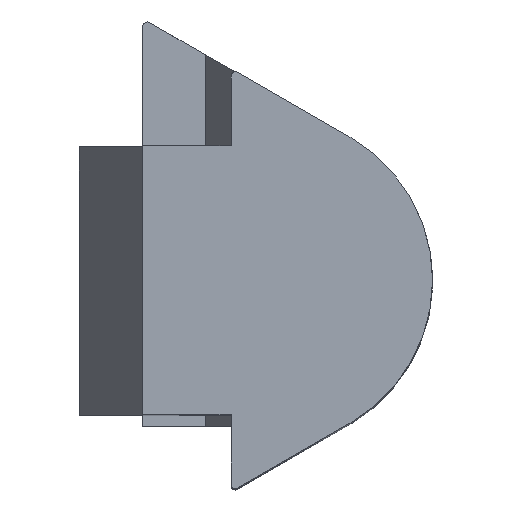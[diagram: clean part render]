
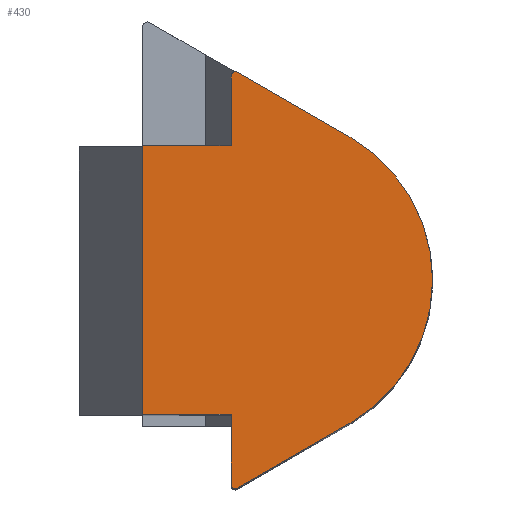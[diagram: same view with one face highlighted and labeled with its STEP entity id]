
A CAD part, top view. The second image highlights one B-rep face of the part: STEP entity #430.
In plain terms, the highlighted planar face has unit normal (0, 0, 1).
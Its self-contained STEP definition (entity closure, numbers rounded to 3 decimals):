
#4 = DIRECTION ( 'NONE',  ( -0.866, -0.5, 0. ) ) ;
#23 = ORIENTED_EDGE ( 'NONE', *, *, #490, .F. ) ;
#28 = LINE ( 'NONE', #186, #461 ) ;
#29 = AXIS2_PLACEMENT_3D ( 'NONE', #381, #360, #355 ) ;
#31 = DIRECTION ( 'NONE',  ( 0., -1., 0. ) ) ;
#33 = DIRECTION ( 'NONE',  ( 0., -1., 0. ) ) ;
#35 = CARTESIAN_POINT ( 'NONE',  ( 2.242, 1.045, -2.686 ) ) ;
#55 = VERTEX_POINT ( 'NONE', #818 ) ;
#66 = AXIS2_PLACEMENT_3D ( 'NONE', #272, #269, #264 ) ;
#73 = ORIENTED_EDGE ( 'NONE', *, *, #546, .F. ) ;
#75 = AXIS2_PLACEMENT_3D ( 'NONE', #684, #641, #633 ) ;
#81 = CARTESIAN_POINT ( 'NONE',  ( 2.306, -2.942, -2.686 ) ) ;
#88 = CARTESIAN_POINT ( 'NONE',  ( 3.958, -2.062, -2.686 ) ) ;
#89 = VECTOR ( 'NONE', #289, 1000. ) ;
#104 = VERTEX_POINT ( 'NONE', #437 ) ;
#109 = CARTESIAN_POINT ( 'NONE',  ( 3.958, -2.062, -2.686 ) ) ;
#111 = DIRECTION ( 'NONE',  ( -1., 0., 0. ) ) ;
#112 = AXIS2_PLACEMENT_3D ( 'NONE', #745, #744, #712 ) ;
#114 = ORIENTED_EDGE ( 'NONE', *, *, #393, .F. ) ;
#117 = AXIS2_PLACEMENT_3D ( 'NONE', #911, #908, #906 ) ;
#128 = CARTESIAN_POINT ( 'NONE',  ( 2.242, -1.045, -2.686 ) ) ;
#132 = CARTESIAN_POINT ( 'NONE',  ( 2.102, 1.937, -2.686 ) ) ;
#139 = AXIS2_PLACEMENT_3D ( 'NONE', #81, #973, #968 ) ;
#141 = CARTESIAN_POINT ( 'NONE',  ( 2.242, 1.937, -2.686 ) ) ;
#156 = DIRECTION ( 'NONE',  ( 0., 1., 0. ) ) ;
#186 = CARTESIAN_POINT ( 'NONE',  ( 0.972, -2.089, -2.686 ) ) ;
#223 = VECTOR ( 'NONE', #33, 1000. ) ;
#224 = ORIENTED_EDGE ( 'NONE', *, *, #370, .F. ) ;
#256 = LINE ( 'NONE', #88, #671 ) ;
#264 = DIRECTION ( 'NONE',  ( -0.5, 0.866, 0. ) ) ;
#267 = CARTESIAN_POINT ( 'NONE',  ( 2.102, -1.937, -2.686 ) ) ;
#269 = DIRECTION ( 'NONE',  ( 0., 0., -1. ) ) ;
#272 = CARTESIAN_POINT ( 'NONE',  ( 2.306, 2.942, -2.686 ) ) ;
#279 = EDGE_LOOP ( 'NONE', ( #515, #224, #73, #543, #462, #114, #333, #821, #23, #579, #930, #374 ) ) ;
#289 = DIRECTION ( 'NONE',  ( 1., 0., 0. ) ) ;
#298 = CIRCLE ( 'NONE', #66, 0.063 ) ;
#299 = LINE ( 'NONE', #128, #701 ) ;
#333 = ORIENTED_EDGE ( 'NONE', *, *, #505, .T. ) ;
#336 = DIRECTION ( 'NONE',  ( 0.866, -0.5, 0. ) ) ;
#341 = EDGE_CURVE ( 'NONE', #392, #765, #576, .T. ) ;
#355 = DIRECTION ( 'NONE',  ( 0.5, 0.866, 0. ) ) ;
#360 = DIRECTION ( 'NONE',  ( 0., 0., -1. ) ) ;
#370 = EDGE_CURVE ( 'NONE', #501, #832, #256, .T. ) ;
#374 = ORIENTED_EDGE ( 'NONE', *, *, #380, .F. ) ;
#380 = EDGE_CURVE ( 'NONE', #519, #411, #839, .T. ) ;
#381 = CARTESIAN_POINT ( 'NONE',  ( 2.767, 0., -2.686 ) ) ;
#389 = FACE_OUTER_BOUND ( 'NONE', #279, .T. ) ;
#392 = VERTEX_POINT ( 'NONE', #431 ) ;
#393 = EDGE_CURVE ( 'NONE', #436, #104, #797, .T. ) ;
#411 = VERTEX_POINT ( 'NONE', #812 ) ;
#417 = CIRCLE ( 'NONE', #112, 0.064 ) ;
#420 = EDGE_CURVE ( 'NONE', #832, #519, #417, .T. ) ;
#430 = ADVANCED_FACE ( 'NONE', ( #389 ), #643, .T. ) ;
#431 = CARTESIAN_POINT ( 'NONE',  ( 2.338, 2.997, -2.686 ) ) ;
#436 = VERTEX_POINT ( 'NONE', #578 ) ;
#437 = CARTESIAN_POINT ( 'NONE',  ( 2.274, 2.997, -2.686 ) ) ;
#461 = VECTOR ( 'NONE', #156, 1000. ) ;
#462 = ORIENTED_EDGE ( 'NONE', *, *, #477, .F. ) ;
#477 = EDGE_CURVE ( 'NONE', #104, #392, #298, .T. ) ;
#490 = EDGE_CURVE ( 'NONE', #682, #55, #28, .T. ) ;
#501 = VERTEX_POINT ( 'NONE', #109 ) ;
#505 = EDGE_CURVE ( 'NONE', #436, #673, #630, .T. ) ;
#515 = ORIENTED_EDGE ( 'NONE', *, *, #420, .F. ) ;
#519 = VERTEX_POINT ( 'NONE', #939 ) ;
#524 = VECTOR ( 'NONE', #111, 1000. ) ;
#543 = ORIENTED_EDGE ( 'NONE', *, *, #341, .F. ) ;
#546 = EDGE_CURVE ( 'NONE', #765, #501, #917, .T. ) ;
#558 = EDGE_CURVE ( 'NONE', #673, #55, #896, .T. ) ;
#562 = EDGE_CURVE ( 'NONE', #682, #949, #743, .T. ) ;
#566 = EDGE_CURVE ( 'NONE', #949, #411, #299, .T. ) ;
#576 = LINE ( 'NONE', #733, #886 ) ;
#578 = CARTESIAN_POINT ( 'NONE',  ( 2.242, 2.942, -2.686 ) ) ;
#579 = ORIENTED_EDGE ( 'NONE', *, *, #562, .T. ) ;
#630 = LINE ( 'NONE', #35, #223 ) ;
#633 = DIRECTION ( 'NONE',  ( 1., 0., 0. ) ) ;
#640 = CARTESIAN_POINT ( 'NONE',  ( 3.958, 2.062, -2.686 ) ) ;
#641 = DIRECTION ( 'NONE',  ( 0., 0., 1. ) ) ;
#643 = PLANE ( 'NONE',  #75 ) ;
#671 = VECTOR ( 'NONE', #4, 1000. ) ;
#673 = VERTEX_POINT ( 'NONE', #141 ) ;
#682 = VERTEX_POINT ( 'NONE', #762 ) ;
#684 = CARTESIAN_POINT ( 'NONE',  ( 2.598, 0., -2.686 ) ) ;
#701 = VECTOR ( 'NONE', #31, 1000. ) ;
#708 = CARTESIAN_POINT ( 'NONE',  ( 2.338, -2.997, -2.686 ) ) ;
#712 = DIRECTION ( 'NONE',  ( -0.5, -0.866, 0. ) ) ;
#733 = CARTESIAN_POINT ( 'NONE',  ( 2.242, 3.052, -2.686 ) ) ;
#743 = LINE ( 'NONE', #267, #89 ) ;
#744 = DIRECTION ( 'NONE',  ( 0., 0., -1. ) ) ;
#745 = CARTESIAN_POINT ( 'NONE',  ( 2.306, -2.942, -2.686 ) ) ;
#762 = CARTESIAN_POINT ( 'NONE',  ( 0.972, -1.937, -2.686 ) ) ;
#765 = VERTEX_POINT ( 'NONE', #640 ) ;
#797 = CIRCLE ( 'NONE', #117, 0.063 ) ;
#812 = CARTESIAN_POINT ( 'NONE',  ( 2.242, -2.942, -2.686 ) ) ;
#818 = CARTESIAN_POINT ( 'NONE',  ( 0.972, 1.937, -2.686 ) ) ;
#821 = ORIENTED_EDGE ( 'NONE', *, *, #558, .T. ) ;
#832 = VERTEX_POINT ( 'NONE', #708 ) ;
#839 = CIRCLE ( 'NONE', #139, 0.064 ) ;
#886 = VECTOR ( 'NONE', #336, 1000. ) ;
#896 = LINE ( 'NONE', #132, #524 ) ;
#906 = DIRECTION ( 'NONE',  ( -0.5, 0.866, 0. ) ) ;
#908 = DIRECTION ( 'NONE',  ( 0., 0., -1. ) ) ;
#911 = CARTESIAN_POINT ( 'NONE',  ( 2.306, 2.942, -2.686 ) ) ;
#914 = CARTESIAN_POINT ( 'NONE',  ( 2.242, -1.937, -2.686 ) ) ;
#917 = CIRCLE ( 'NONE', #29, 2.381 ) ;
#930 = ORIENTED_EDGE ( 'NONE', *, *, #566, .T. ) ;
#939 = CARTESIAN_POINT ( 'NONE',  ( 2.274, -2.997, -2.686 ) ) ;
#949 = VERTEX_POINT ( 'NONE', #914 ) ;
#968 = DIRECTION ( 'NONE',  ( -0.5, -0.866, 0. ) ) ;
#973 = DIRECTION ( 'NONE',  ( 0., 0., -1. ) ) ;
